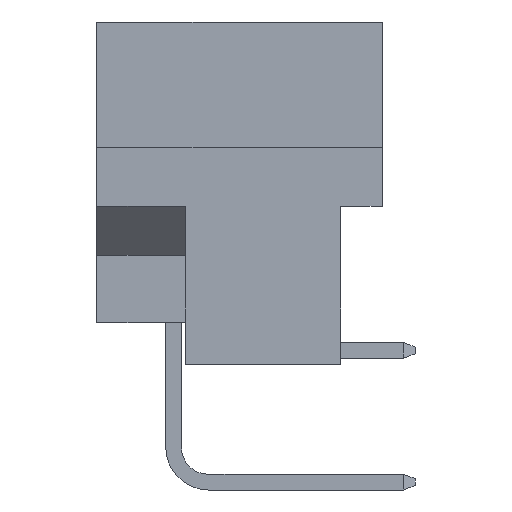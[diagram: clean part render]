
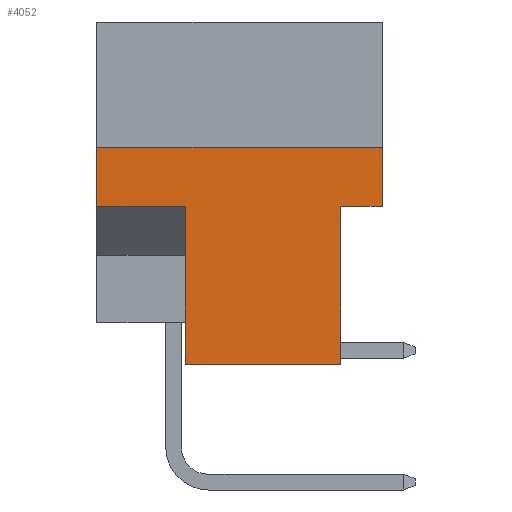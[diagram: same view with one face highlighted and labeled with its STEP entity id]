
A CAD part, left-side view. The second image highlights one B-rep face of the part: STEP entity #4052.
In plain terms, the highlighted planar face has unit normal (-1, 0, 0).
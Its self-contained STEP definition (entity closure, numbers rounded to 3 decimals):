
#314 = VERTEX_POINT ( 'NONE', #7642 ) ;
#388 = ORIENTED_EDGE ( 'NONE', *, *, #9128, .F. ) ;
#627 = DIRECTION ( 'NONE',  ( 0., -1., 0. ) ) ;
#706 = CARTESIAN_POINT ( 'NONE',  ( 0., 7.597, -13.2 ) ) ;
#786 = VERTEX_POINT ( 'NONE', #8202 ) ;
#976 = EDGE_CURVE ( 'NONE', #7184, #2694, #7909, .T. ) ;
#995 = ORIENTED_EDGE ( 'NONE', *, *, #976, .F. ) ;
#1033 = DIRECTION ( 'NONE',  ( 0., 1., 0. ) ) ;
#1064 = EDGE_CURVE ( 'NONE', #6983, #7184, #7589, .T. ) ;
#1473 = AXIS2_PLACEMENT_3D ( 'NONE', #5200, #8163, #1639 ) ;
#1477 = CARTESIAN_POINT ( 'NONE',  ( 0., 1.6, 46.912 ) ) ;
#1639 = DIRECTION ( 'NONE',  ( 0., 0., -1. ) ) ;
#1687 = EDGE_LOOP ( 'NONE', ( #995, #7631, #1920, #2928, #388, #3554, #1957, #7820 ) ) ;
#1707 = DIRECTION ( 'NONE',  ( 0., 1., 0. ) ) ;
#1920 = ORIENTED_EDGE ( 'NONE', *, *, #8480, .T. ) ;
#1957 = ORIENTED_EDGE ( 'NONE', *, *, #6020, .F. ) ;
#2315 = VECTOR ( 'NONE', #5097, 1000. ) ;
#2599 = VERTEX_POINT ( 'NONE', #706 ) ;
#2664 = VECTOR ( 'NONE', #8382, 1000. ) ;
#2694 = VERTEX_POINT ( 'NONE', #2808 ) ;
#2750 = CARTESIAN_POINT ( 'NONE',  ( 0., 7.597, -13.2 ) ) ;
#2808 = CARTESIAN_POINT ( 'NONE',  ( 0., 1.6, -13.2 ) ) ;
#2901 = CARTESIAN_POINT ( 'NONE',  ( 0., 10.998, 0. ) ) ;
#2928 = ORIENTED_EDGE ( 'NONE', *, *, #3212, .F. ) ;
#2929 = CARTESIAN_POINT ( 'NONE',  ( 0., 10.998, -4.826 ) ) ;
#3212 = EDGE_CURVE ( 'NONE', #314, #4634, #5843, .T. ) ;
#3339 = CARTESIAN_POINT ( 'NONE',  ( 0., 10.998, -13.2 ) ) ;
#3554 = ORIENTED_EDGE ( 'NONE', *, *, #4029, .F. ) ;
#3569 = VECTOR ( 'NONE', #627, 1000. ) ;
#3832 = FACE_OUTER_BOUND ( 'NONE', #1687, .T. ) ;
#3866 = VECTOR ( 'NONE', #1033, 1000. ) ;
#4008 = CARTESIAN_POINT ( 'NONE',  ( 0., 0., -7.112 ) ) ;
#4029 = EDGE_CURVE ( 'NONE', #7581, #786, #6750, .T. ) ;
#4052 = ADVANCED_FACE ( 'NONE', ( #3832 ), #4542, .F. ) ;
#4337 = DIRECTION ( 'NONE',  ( 0., 0., -1. ) ) ;
#4542 = PLANE ( 'NONE',  #1473 ) ;
#4634 = VERTEX_POINT ( 'NONE', #5567 ) ;
#5067 = LINE ( 'NONE', #2901, #8662 ) ;
#5097 = DIRECTION ( 'NONE',  ( 0., -1., 0. ) ) ;
#5200 = CARTESIAN_POINT ( 'NONE',  ( 0., 10.998, 0. ) ) ;
#5259 = CARTESIAN_POINT ( 'NONE',  ( 0., 7.597, -7.112 ) ) ;
#5567 = CARTESIAN_POINT ( 'NONE',  ( 0., 0., -4.826 ) ) ;
#5609 = CARTESIAN_POINT ( 'NONE',  ( 0., 0., 0. ) ) ;
#5698 = VECTOR ( 'NONE', #1707, 1000. ) ;
#5843 = LINE ( 'NONE', #2929, #2315 ) ;
#6020 = EDGE_CURVE ( 'NONE', #2599, #7581, #9196, .T. ) ;
#6149 = VECTOR ( 'NONE', #4337, 1000. ) ;
#6750 = LINE ( 'NONE', #8019, #3866 ) ;
#6983 = VERTEX_POINT ( 'NONE', #7160 ) ;
#7012 = LINE ( 'NONE', #3339, #3569 ) ;
#7066 = LINE ( 'NONE', #5609, #2664 ) ;
#7160 = CARTESIAN_POINT ( 'NONE',  ( 0., 0., -7.112 ) ) ;
#7184 = VERTEX_POINT ( 'NONE', #8887 ) ;
#7581 = VERTEX_POINT ( 'NONE', #5259 ) ;
#7589 = LINE ( 'NONE', #4008, #5698 ) ;
#7631 = ORIENTED_EDGE ( 'NONE', *, *, #1064, .F. ) ;
#7642 = CARTESIAN_POINT ( 'NONE',  ( 0., 10.998, -4.826 ) ) ;
#7820 = ORIENTED_EDGE ( 'NONE', *, *, #9018, .T. ) ;
#7869 = DIRECTION ( 'NONE',  ( 0., 0., 1. ) ) ;
#7909 = LINE ( 'NONE', #1477, #6149 ) ;
#8019 = CARTESIAN_POINT ( 'NONE',  ( 0., 7.597, -7.112 ) ) ;
#8163 = DIRECTION ( 'NONE',  ( 1., 0., 0. ) ) ;
#8202 = CARTESIAN_POINT ( 'NONE',  ( 0., 10.998, -7.112 ) ) ;
#8382 = DIRECTION ( 'NONE',  ( 0., 0., 1. ) ) ;
#8480 = EDGE_CURVE ( 'NONE', #6983, #4634, #7066, .T. ) ;
#8637 = DIRECTION ( 'NONE',  ( 0., 0., 1. ) ) ;
#8662 = VECTOR ( 'NONE', #8637, 1000. ) ;
#8887 = CARTESIAN_POINT ( 'NONE',  ( 0., 1.6, -7.112 ) ) ;
#9018 = EDGE_CURVE ( 'NONE', #2599, #2694, #7012, .T. ) ;
#9108 = VECTOR ( 'NONE', #7869, 1000. ) ;
#9128 = EDGE_CURVE ( 'NONE', #786, #314, #5067, .T. ) ;
#9196 = LINE ( 'NONE', #2750, #9108 ) ;
